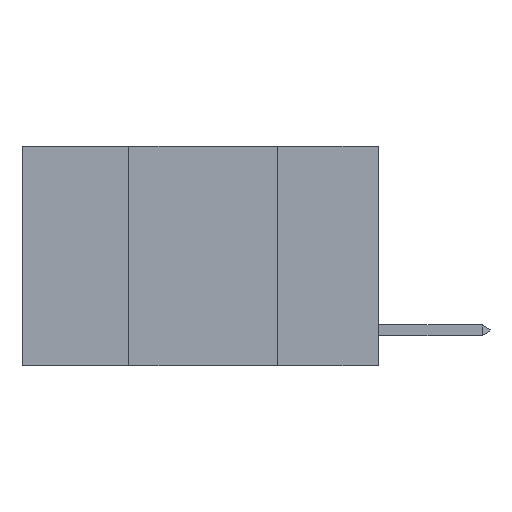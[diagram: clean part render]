
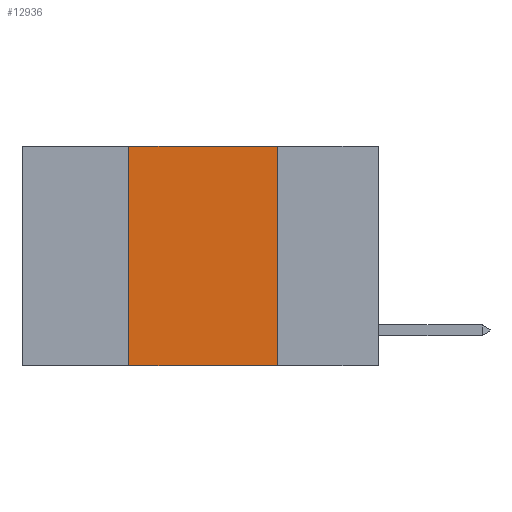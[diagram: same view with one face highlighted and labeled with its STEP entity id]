
A CAD part, left-side view. The second image highlights one B-rep face of the part: STEP entity #12936.
In plain terms, the highlighted planar face has unit normal (-1, 0, 0).
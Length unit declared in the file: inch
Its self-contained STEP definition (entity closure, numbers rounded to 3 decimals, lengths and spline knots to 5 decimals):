
#172 = FACE_OUTER_BOUND ( 'NONE', #2795, .T. ) ;
#390 = VERTEX_POINT ( 'NONE', #17386 ) ;
#559 = EDGE_CURVE ( 'NONE', #11851, #390, #839, .T. ) ;
#839 = LINE ( 'NONE', #5453, #3651 ) ;
#1308 = CARTESIAN_POINT ( 'NONE',  ( 0., 0.42, -0.37 ) ) ;
#1674 = CARTESIAN_POINT ( 'NONE',  ( 0., 0.42, 0. ) ) ;
#1824 = VERTEX_POINT ( 'NONE', #1308 ) ;
#2731 = ORIENTED_EDGE ( 'NONE', *, *, #559, .F. ) ;
#2795 = EDGE_LOOP ( 'NONE', ( #14469, #2731, #16826, #6933 ) ) ;
#3203 = VECTOR ( 'NONE', #9128, 39.37008 ) ;
#3411 = LINE ( 'NONE', #10841, #17075 ) ;
#3437 = EDGE_CURVE ( 'NONE', #1824, #17589, #3411, .T. ) ;
#3651 = VECTOR ( 'NONE', #9550, 39.37008 ) ;
#3895 = EDGE_CURVE ( 'NONE', #1824, #11851, #14131, .T. ) ;
#4336 = EDGE_CURVE ( 'NONE', #390, #17589, #9587, .T. ) ;
#5327 = DIRECTION ( 'NONE',  ( 0., 0., -1. ) ) ;
#5453 = CARTESIAN_POINT ( 'NONE',  ( 0., 0.6, 0. ) ) ;
#6933 = ORIENTED_EDGE ( 'NONE', *, *, #3437, .T. ) ;
#8120 = DIRECTION ( 'NONE',  ( 0., -1., 0. ) ) ;
#9128 = DIRECTION ( 'NONE',  ( 0., 0., 1. ) ) ;
#9550 = DIRECTION ( 'NONE',  ( 0., -1., 0. ) ) ;
#9587 = LINE ( 'NONE', #10113, #10442 ) ;
#10022 = AXIS2_PLACEMENT_3D ( 'NONE', #12116, #13514, #5327 ) ;
#10113 = CARTESIAN_POINT ( 'NONE',  ( 0., 0.17, 0. ) ) ;
#10442 = VECTOR ( 'NONE', #14273, 39.37008 ) ;
#10841 = CARTESIAN_POINT ( 'NONE',  ( 0., 0.6, -0.37 ) ) ;
#11851 = VERTEX_POINT ( 'NONE', #1674 ) ;
#11864 = CARTESIAN_POINT ( 'NONE',  ( 0., 0.42, 0. ) ) ;
#12116 = CARTESIAN_POINT ( 'NONE',  ( 0., 0.6, 0. ) ) ;
#12936 = ADVANCED_FACE ( 'NONE', ( #172 ), #14842, .F. ) ;
#13514 = DIRECTION ( 'NONE',  ( 1., 0., 0. ) ) ;
#13605 = CARTESIAN_POINT ( 'NONE',  ( 0., 0.17, -0.37 ) ) ;
#14131 = LINE ( 'NONE', #11864, #3203 ) ;
#14273 = DIRECTION ( 'NONE',  ( 0., 0., -1. ) ) ;
#14469 = ORIENTED_EDGE ( 'NONE', *, *, #4336, .F. ) ;
#14842 = PLANE ( 'NONE',  #10022 ) ;
#16826 = ORIENTED_EDGE ( 'NONE', *, *, #3895, .F. ) ;
#17075 = VECTOR ( 'NONE', #8120, 39.37008 ) ;
#17386 = CARTESIAN_POINT ( 'NONE',  ( 0., 0.17, 0. ) ) ;
#17589 = VERTEX_POINT ( 'NONE', #13605 ) ;
